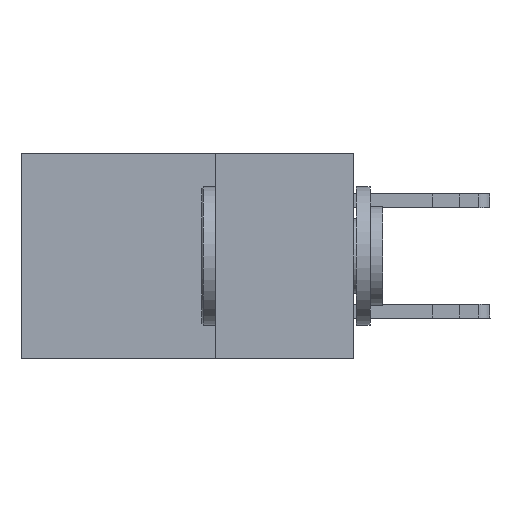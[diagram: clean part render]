
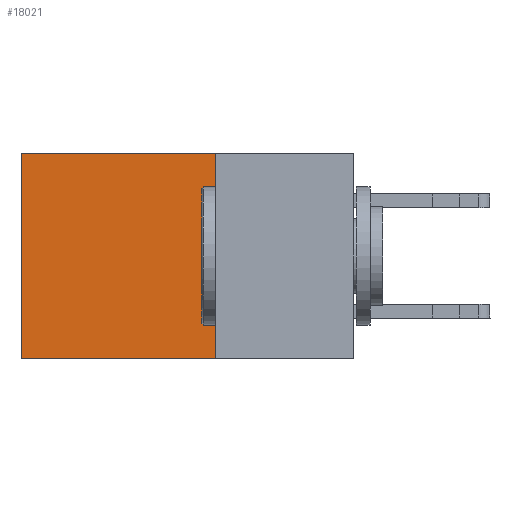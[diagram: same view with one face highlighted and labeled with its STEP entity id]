
A CAD part, left-side view. The second image highlights one B-rep face of the part: STEP entity #18021.
In plain terms, the highlighted planar face has unit normal (-1, 0, 0).
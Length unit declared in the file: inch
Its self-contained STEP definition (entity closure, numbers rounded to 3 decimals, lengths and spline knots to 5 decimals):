
#354 = VECTOR ( 'NONE', #16856, 39.37008 ) ;
#1234 = LINE ( 'NONE', #1296, #1562 ) ;
#1296 = CARTESIAN_POINT ( 'NONE',  ( 0.2875, 0.25, 0. ) ) ;
#1562 = VECTOR ( 'NONE', #25336, 39.37008 ) ;
#2091 = LINE ( 'NONE', #11565, #13043 ) ;
#2383 = CARTESIAN_POINT ( 'NONE',  ( 0.2875, 0.25, -0.37 ) ) ;
#2462 = VERTEX_POINT ( 'NONE', #19274 ) ;
#3461 = ORIENTED_EDGE ( 'NONE', *, *, #10739, .T. ) ;
#3869 = EDGE_CURVE ( 'NONE', #23318, #2462, #2091, .T. ) ;
#4550 = FACE_OUTER_BOUND ( 'NONE', #15719, .T. ) ;
#6015 = CARTESIAN_POINT ( 'NONE',  ( 0.2875, 0.25, 0. ) ) ;
#7443 = ORIENTED_EDGE ( 'NONE', *, *, #3869, .T. ) ;
#7740 = VECTOR ( 'NONE', #24319, 39.37008 ) ;
#10054 = CARTESIAN_POINT ( 'NONE',  ( 0.2875, 0.6, -0.37 ) ) ;
#10514 = ORIENTED_EDGE ( 'NONE', *, *, #12347, .F. ) ;
#10739 = EDGE_CURVE ( 'NONE', #2462, #20712, #11934, .T. ) ;
#11565 = CARTESIAN_POINT ( 'NONE',  ( 0.2875, 0.25, 0. ) ) ;
#11886 = CARTESIAN_POINT ( 'NONE',  ( 0.2875, 0.25, 0. ) ) ;
#11934 = LINE ( 'NONE', #21107, #354 ) ;
#12347 = EDGE_CURVE ( 'NONE', #18452, #20712, #25282, .T. ) ;
#13043 = VECTOR ( 'NONE', #22246, 39.37008 ) ;
#13275 = EDGE_CURVE ( 'NONE', #23318, #18452, #1234, .T. ) ;
#15719 = EDGE_LOOP ( 'NONE', ( #3461, #10514, #20830, #7443 ) ) ;
#16758 = DIRECTION ( 'NONE',  ( 1., 0., 0. ) ) ;
#16856 = DIRECTION ( 'NONE',  ( 0., 0., -1. ) ) ;
#18021 = ADVANCED_FACE ( 'NONE', ( #4550 ), #27807, .F. ) ;
#18452 = VERTEX_POINT ( 'NONE', #20212 ) ;
#19068 = DIRECTION ( 'NONE',  ( 0., 0., -1. ) ) ;
#19274 = CARTESIAN_POINT ( 'NONE',  ( 0.2875, 0.6, 0. ) ) ;
#20212 = CARTESIAN_POINT ( 'NONE',  ( 0.2875, 0.25, -0.37 ) ) ;
#20712 = VERTEX_POINT ( 'NONE', #10054 ) ;
#20830 = ORIENTED_EDGE ( 'NONE', *, *, #13275, .F. ) ;
#21107 = CARTESIAN_POINT ( 'NONE',  ( 0.2875, 0.6, 0. ) ) ;
#21349 = AXIS2_PLACEMENT_3D ( 'NONE', #6015, #16758, #19068 ) ;
#22246 = DIRECTION ( 'NONE',  ( 0., 1., 0. ) ) ;
#23318 = VERTEX_POINT ( 'NONE', #11886 ) ;
#24319 = DIRECTION ( 'NONE',  ( 0., 1., 0. ) ) ;
#25282 = LINE ( 'NONE', #2383, #7740 ) ;
#25336 = DIRECTION ( 'NONE',  ( 0., 0., -1. ) ) ;
#27807 = PLANE ( 'NONE',  #21349 ) ;
